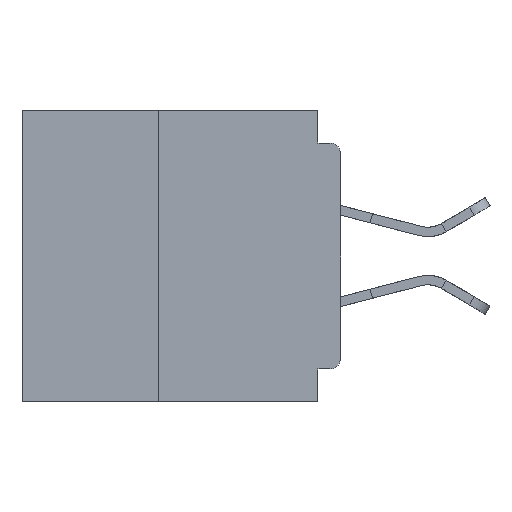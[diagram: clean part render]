
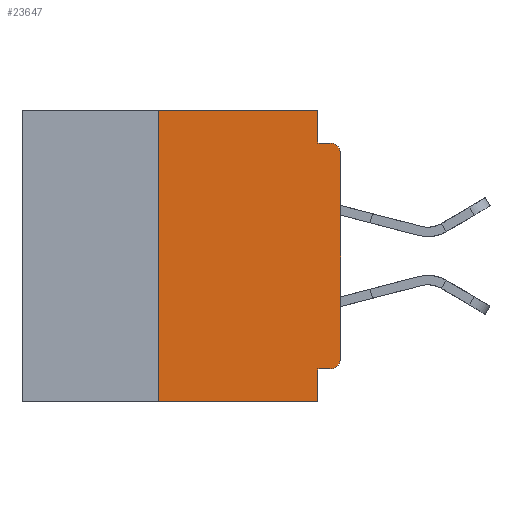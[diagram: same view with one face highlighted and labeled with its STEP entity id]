
A CAD part, left-side view. The second image highlights one B-rep face of the part: STEP entity #23647.
In plain terms, the highlighted planar face has unit normal (-1, 0, 0).
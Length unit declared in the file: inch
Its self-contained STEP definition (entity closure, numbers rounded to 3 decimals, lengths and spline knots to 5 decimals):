
#481 = CARTESIAN_POINT ( 'NONE',  ( 0., 0.015, -0.355 ) ) ;
#555 = CARTESIAN_POINT ( 'NONE',  ( 0., 0.015, -0.045 ) ) ;
#3266 = VERTEX_POINT ( 'NONE', #14551 ) ;
#3540 = DIRECTION ( 'NONE',  ( 0., -1., 0. ) ) ;
#4025 = ORIENTED_EDGE ( 'NONE', *, *, #49165, .T. ) ;
#4096 = ORIENTED_EDGE ( 'NONE', *, *, #28266, .F. ) ;
#4618 = ORIENTED_EDGE ( 'NONE', *, *, #34860, .F. ) ;
#4749 = CARTESIAN_POINT ( 'NONE',  ( 0., 0.25, -0.4 ) ) ;
#6588 = DIRECTION ( 'NONE',  ( 0., 0., 1. ) ) ;
#7499 = CIRCLE ( 'NONE', #29720, 0.015 ) ;
#7582 = CARTESIAN_POINT ( 'NONE',  ( 0., 0.015, -0.34 ) ) ;
#8536 = EDGE_CURVE ( 'NONE', #3266, #14370, #39854, .T. ) ;
#8681 = DIRECTION ( 'NONE',  ( 0., 0., 1. ) ) ;
#9980 = ORIENTED_EDGE ( 'NONE', *, *, #44176, .T. ) ;
#10118 = LINE ( 'NONE', #39482, #29665 ) ;
#10389 = DIRECTION ( 'NONE',  ( 0., 0., -1. ) ) ;
#10627 = CARTESIAN_POINT ( 'NONE',  ( 0., 0.015, -0.06 ) ) ;
#10834 = AXIS2_PLACEMENT_3D ( 'NONE', #7582, #34826, #11491 ) ;
#11226 = CARTESIAN_POINT ( 'NONE',  ( 0., 0.437, -0.4 ) ) ;
#11491 = DIRECTION ( 'NONE',  ( 0., 0., -1. ) ) ;
#11771 = ORIENTED_EDGE ( 'NONE', *, *, #46409, .F. ) ;
#12099 = LINE ( 'NONE', #30101, #14606 ) ;
#12267 = VERTEX_POINT ( 'NONE', #15379 ) ;
#12547 = VECTOR ( 'NONE', #3540, 39.37008 ) ;
#13805 = LINE ( 'NONE', #42286, #43513 ) ;
#14370 = VERTEX_POINT ( 'NONE', #26394 ) ;
#14397 = ORIENTED_EDGE ( 'NONE', *, *, #19054, .T. ) ;
#14551 = CARTESIAN_POINT ( 'NONE',  ( 0., 0.031, -0.355 ) ) ;
#14588 = DIRECTION ( 'NONE',  ( 0., 0., -1. ) ) ;
#14606 = VECTOR ( 'NONE', #6588, 39.37008 ) ;
#15379 = CARTESIAN_POINT ( 'NONE',  ( 0., 0., -0.06 ) ) ;
#15708 = CARTESIAN_POINT ( 'NONE',  ( 0., 0.437, 0. ) ) ;
#15871 = DIRECTION ( 'NONE',  ( 0., 0., -1. ) ) ;
#16249 = VECTOR ( 'NONE', #50203, 39.37008 ) ;
#18888 = CARTESIAN_POINT ( 'NONE',  ( 0., 0.031, -0.045 ) ) ;
#19054 = EDGE_CURVE ( 'NONE', #12267, #39484, #7499, .T. ) ;
#19290 = CARTESIAN_POINT ( 'NONE',  ( 0., 0., -0.045 ) ) ;
#19820 = LINE ( 'NONE', #4749, #38084 ) ;
#22928 = LINE ( 'NONE', #11226, #12547 ) ;
#23061 = ORIENTED_EDGE ( 'NONE', *, *, #34869, .T. ) ;
#23546 = FACE_OUTER_BOUND ( 'NONE', #45588, .T. ) ;
#23577 = ORIENTED_EDGE ( 'NONE', *, *, #8536, .F. ) ;
#23647 = ADVANCED_FACE ( 'NONE', ( #23546 ), #31363, .F. ) ;
#24388 = ORIENTED_EDGE ( 'NONE', *, *, #46273, .F. ) ;
#26394 = CARTESIAN_POINT ( 'NONE',  ( 0., 0.031, -0.4 ) ) ;
#27856 = LINE ( 'NONE', #19290, #16249 ) ;
#28266 = EDGE_CURVE ( 'NONE', #34567, #49754, #19820, .T. ) ;
#29665 = VECTOR ( 'NONE', #43341, 39.37008 ) ;
#29720 = AXIS2_PLACEMENT_3D ( 'NONE', #10627, #37837, #14588 ) ;
#30056 = VERTEX_POINT ( 'NONE', #481 ) ;
#30101 = CARTESIAN_POINT ( 'NONE',  ( 0., 0., 0. ) ) ;
#30619 = CARTESIAN_POINT ( 'NONE',  ( 0., 0., -0.34 ) ) ;
#31363 = PLANE ( 'NONE',  #40207 ) ;
#34567 = VERTEX_POINT ( 'NONE', #48339 ) ;
#34826 = DIRECTION ( 'NONE',  ( -1., 0., 0. ) ) ;
#34860 = EDGE_CURVE ( 'NONE', #49987, #48494, #13805, .T. ) ;
#34869 = EDGE_CURVE ( 'NONE', #34567, #14370, #22928, .T. ) ;
#36185 = EDGE_CURVE ( 'NONE', #49754, #49987, #42179, .T. ) ;
#37090 = ORIENTED_EDGE ( 'NONE', *, *, #36185, .F. ) ;
#37597 = CARTESIAN_POINT ( 'NONE',  ( 0., 0.031, -0.4 ) ) ;
#37837 = DIRECTION ( 'NONE',  ( -1., 0., 0. ) ) ;
#38084 = VECTOR ( 'NONE', #8681, 39.37008 ) ;
#38805 = DIRECTION ( 'NONE',  ( 0., -1., 0. ) ) ;
#39108 = DIRECTION ( 'NONE',  ( 1., 0., 0. ) ) ;
#39482 = CARTESIAN_POINT ( 'NONE',  ( 0., 0., -0.355 ) ) ;
#39484 = VERTEX_POINT ( 'NONE', #555 ) ;
#39854 = LINE ( 'NONE', #37597, #48823 ) ;
#40207 = AXIS2_PLACEMENT_3D ( 'NONE', #15708, #39108, #15871 ) ;
#40989 = VECTOR ( 'NONE', #38805, 39.37008 ) ;
#42179 = LINE ( 'NONE', #46345, #40989 ) ;
#42286 = CARTESIAN_POINT ( 'NONE',  ( 0., 0.031, 0. ) ) ;
#43341 = DIRECTION ( 'NONE',  ( 0., 1., 0. ) ) ;
#43513 = VECTOR ( 'NONE', #46144, 39.37008 ) ;
#44176 = EDGE_CURVE ( 'NONE', #44220, #12267, #12099, .T. ) ;
#44220 = VERTEX_POINT ( 'NONE', #30619 ) ;
#45588 = EDGE_LOOP ( 'NONE', ( #9980, #14397, #24388, #4618, #37090, #4096, #23061, #23577, #11771, #4025 ) ) ;
#46017 = CARTESIAN_POINT ( 'NONE',  ( 0., 0.25, 0. ) ) ;
#46144 = DIRECTION ( 'NONE',  ( 0., 0., -1. ) ) ;
#46273 = EDGE_CURVE ( 'NONE', #48494, #39484, #27856, .T. ) ;
#46345 = CARTESIAN_POINT ( 'NONE',  ( 0., 0.437, 0. ) ) ;
#46409 = EDGE_CURVE ( 'NONE', #30056, #3266, #10118, .T. ) ;
#47485 = CARTESIAN_POINT ( 'NONE',  ( 0., 0.031, 0. ) ) ;
#48163 = CIRCLE ( 'NONE', #10834, 0.015 ) ;
#48339 = CARTESIAN_POINT ( 'NONE',  ( 0., 0.25, -0.4 ) ) ;
#48494 = VERTEX_POINT ( 'NONE', #18888 ) ;
#48823 = VECTOR ( 'NONE', #10389, 39.37008 ) ;
#49165 = EDGE_CURVE ( 'NONE', #30056, #44220, #48163, .T. ) ;
#49754 = VERTEX_POINT ( 'NONE', #46017 ) ;
#49987 = VERTEX_POINT ( 'NONE', #47485 ) ;
#50203 = DIRECTION ( 'NONE',  ( 0., -1., 0. ) ) ;
